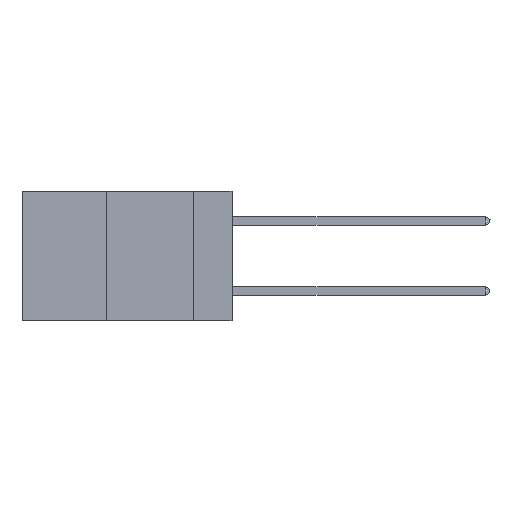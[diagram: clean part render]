
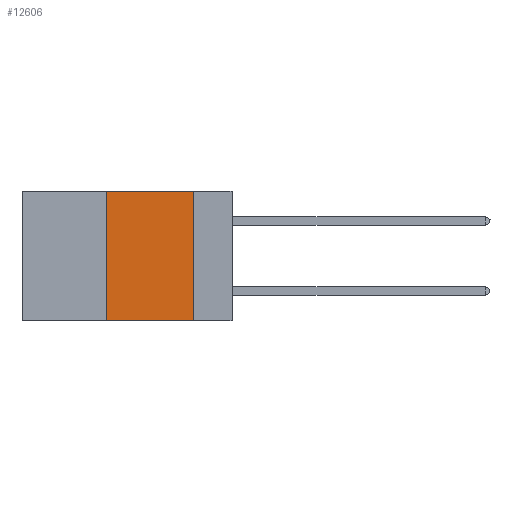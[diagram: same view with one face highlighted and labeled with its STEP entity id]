
A CAD part, left-side view. The second image highlights one B-rep face of the part: STEP entity #12606.
In plain terms, the highlighted planar face has unit normal (-1, 0, 0).
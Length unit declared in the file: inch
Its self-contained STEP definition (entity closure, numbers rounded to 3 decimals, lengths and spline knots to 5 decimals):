
#53 = FACE_OUTER_BOUND ( 'NONE', #3473, .T. ) ;
#234 = DIRECTION ( 'NONE',  ( 0., 0., 1. ) ) ;
#623 = DIRECTION ( 'NONE',  ( 0., -1., 0. ) ) ;
#1765 = CARTESIAN_POINT ( 'NONE',  ( 0., 0.36, -0.37 ) ) ;
#1905 = DIRECTION ( 'NONE',  ( 0., 0., -1. ) ) ;
#2072 = CARTESIAN_POINT ( 'NONE',  ( 0., 0.11, 0. ) ) ;
#2113 = VERTEX_POINT ( 'NONE', #1765 ) ;
#2374 = ORIENTED_EDGE ( 'NONE', *, *, #5745, .F. ) ;
#3473 = EDGE_LOOP ( 'NONE', ( #10803, #2374, #16421, #9072 ) ) ;
#3611 = VECTOR ( 'NONE', #20269, 39.37008 ) ;
#3933 = EDGE_CURVE ( 'NONE', #2113, #26791, #28278, .T. ) ;
#4027 = CARTESIAN_POINT ( 'NONE',  ( 0., 0.6, 0. ) ) ;
#4481 = CARTESIAN_POINT ( 'NONE',  ( 0., 0.6, 0. ) ) ;
#4730 = CARTESIAN_POINT ( 'NONE',  ( 0., 0.11, -0.37 ) ) ;
#5306 = LINE ( 'NONE', #2072, #20200 ) ;
#5745 = EDGE_CURVE ( 'NONE', #26791, #11418, #6755, .T. ) ;
#6755 = LINE ( 'NONE', #4481, #3611 ) ;
#8423 = DIRECTION ( 'NONE',  ( 1., 0., 0. ) ) ;
#9072 = ORIENTED_EDGE ( 'NONE', *, *, #23309, .T. ) ;
#9404 = VECTOR ( 'NONE', #623, 39.37008 ) ;
#10803 = ORIENTED_EDGE ( 'NONE', *, *, #16535, .F. ) ;
#11418 = VERTEX_POINT ( 'NONE', #17575 ) ;
#12606 = ADVANCED_FACE ( 'NONE', ( #53 ), #26129, .F. ) ;
#13557 = CARTESIAN_POINT ( 'NONE',  ( 0., 0.36, 0. ) ) ;
#13762 = CARTESIAN_POINT ( 'NONE',  ( 0., 0.6, -0.37 ) ) ;
#15870 = VERTEX_POINT ( 'NONE', #4730 ) ;
#16029 = DIRECTION ( 'NONE',  ( 0., 0., -1. ) ) ;
#16421 = ORIENTED_EDGE ( 'NONE', *, *, #3933, .F. ) ;
#16535 = EDGE_CURVE ( 'NONE', #11418, #15870, #5306, .T. ) ;
#17575 = CARTESIAN_POINT ( 'NONE',  ( 0., 0.11, 0. ) ) ;
#20200 = VECTOR ( 'NONE', #16029, 39.37008 ) ;
#20269 = DIRECTION ( 'NONE',  ( 0., -1., 0. ) ) ;
#21195 = LINE ( 'NONE', #13762, #9404 ) ;
#22433 = VECTOR ( 'NONE', #234, 39.37008 ) ;
#23309 = EDGE_CURVE ( 'NONE', #2113, #15870, #21195, .T. ) ;
#23909 = CARTESIAN_POINT ( 'NONE',  ( 0., 0.36, 0. ) ) ;
#24614 = AXIS2_PLACEMENT_3D ( 'NONE', #4027, #8423, #1905 ) ;
#26129 = PLANE ( 'NONE',  #24614 ) ;
#26791 = VERTEX_POINT ( 'NONE', #23909 ) ;
#28278 = LINE ( 'NONE', #13557, #22433 ) ;
